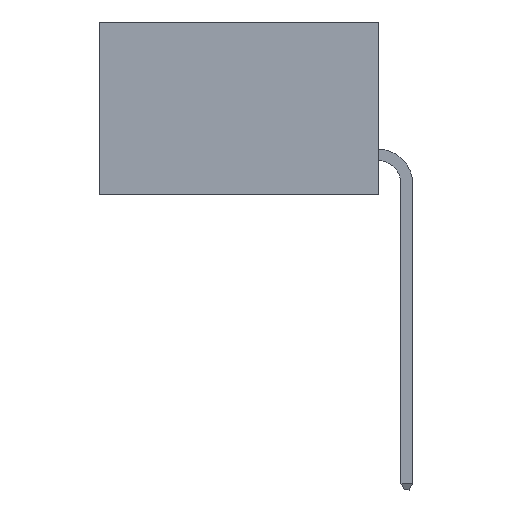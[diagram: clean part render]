
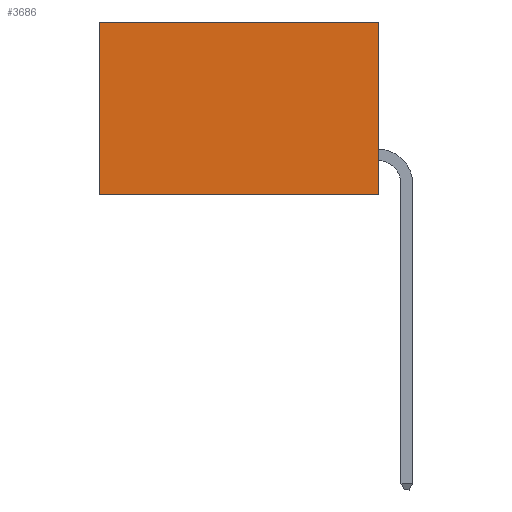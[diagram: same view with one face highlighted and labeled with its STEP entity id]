
A CAD part, left-side view. The second image highlights one B-rep face of the part: STEP entity #3686.
In plain terms, the highlighted planar face has unit normal (-1, 0, 0).
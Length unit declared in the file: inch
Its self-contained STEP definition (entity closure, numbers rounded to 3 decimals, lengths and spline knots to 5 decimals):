
#314 = DIRECTION ( 'NONE',  ( 0., 1., 0. ) ) ;
#648 = ORIENTED_EDGE ( 'NONE', *, *, #13417, .T. ) ;
#1342 = VERTEX_POINT ( 'NONE', #10155 ) ;
#1386 = ORIENTED_EDGE ( 'NONE', *, *, #16828, .F. ) ;
#2126 = LINE ( 'NONE', #27827, #26265 ) ;
#2852 = CARTESIAN_POINT ( 'NONE',  ( 0.298, 0.6, 0. ) ) ;
#3366 = DIRECTION ( 'NONE',  ( 0., 1., 0. ) ) ;
#3686 = ADVANCED_FACE ( 'NONE', ( #29130 ), #26288, .F. ) ;
#7984 = AXIS2_PLACEMENT_3D ( 'NONE', #26261, #26176, #25672 ) ;
#8108 = EDGE_CURVE ( 'NONE', #19871, #15584, #24253, .T. ) ;
#9119 = ORIENTED_EDGE ( 'NONE', *, *, #28851, .F. ) ;
#10155 = CARTESIAN_POINT ( 'NONE',  ( 0.298, 0., 0. ) ) ;
#10299 = CARTESIAN_POINT ( 'NONE',  ( 0.298, 0., -0.37 ) ) ;
#11303 = VECTOR ( 'NONE', #314, 39.37008 ) ;
#12058 = VECTOR ( 'NONE', #25289, 39.37008 ) ;
#13417 = EDGE_CURVE ( 'NONE', #1342, #19871, #24259, .T. ) ;
#13999 = CARTESIAN_POINT ( 'NONE',  ( 0.298, 0., -0.37 ) ) ;
#15584 = VERTEX_POINT ( 'NONE', #29880 ) ;
#16828 = EDGE_CURVE ( 'NONE', #20634, #15584, #26664, .T. ) ;
#16950 = ORIENTED_EDGE ( 'NONE', *, *, #8108, .T. ) ;
#18232 = DIRECTION ( 'NONE',  ( 0., 0., -1. ) ) ;
#19459 = VECTOR ( 'NONE', #3366, 39.37008 ) ;
#19871 = VERTEX_POINT ( 'NONE', #29192 ) ;
#20634 = VERTEX_POINT ( 'NONE', #13999 ) ;
#24019 = EDGE_LOOP ( 'NONE', ( #16950, #1386, #9119, #648 ) ) ;
#24253 = LINE ( 'NONE', #2852, #12058 ) ;
#24259 = LINE ( 'NONE', #29102, #11303 ) ;
#25289 = DIRECTION ( 'NONE',  ( 0., 0., -1. ) ) ;
#25672 = DIRECTION ( 'NONE',  ( 0., 0., -1. ) ) ;
#26176 = DIRECTION ( 'NONE',  ( 1., 0., 0. ) ) ;
#26261 = CARTESIAN_POINT ( 'NONE',  ( 0.298, 0., 0. ) ) ;
#26265 = VECTOR ( 'NONE', #18232, 39.37008 ) ;
#26288 = PLANE ( 'NONE',  #7984 ) ;
#26664 = LINE ( 'NONE', #10299, #19459 ) ;
#27827 = CARTESIAN_POINT ( 'NONE',  ( 0.298, 0., 0. ) ) ;
#28851 = EDGE_CURVE ( 'NONE', #1342, #20634, #2126, .T. ) ;
#29102 = CARTESIAN_POINT ( 'NONE',  ( 0.298, 0., 0. ) ) ;
#29130 = FACE_OUTER_BOUND ( 'NONE', #24019, .T. ) ;
#29192 = CARTESIAN_POINT ( 'NONE',  ( 0.298, 0.6, 0. ) ) ;
#29880 = CARTESIAN_POINT ( 'NONE',  ( 0.298, 0.6, -0.37 ) ) ;
